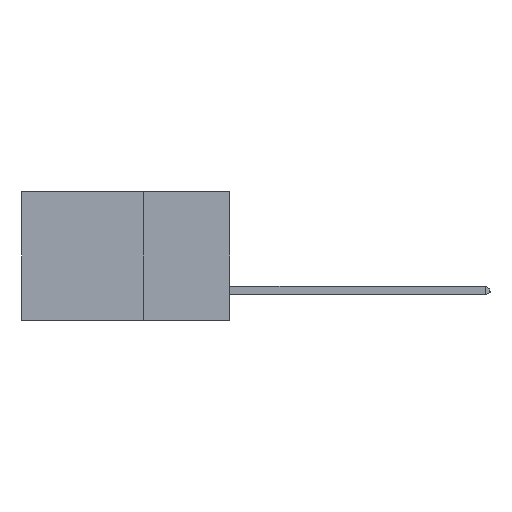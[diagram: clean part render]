
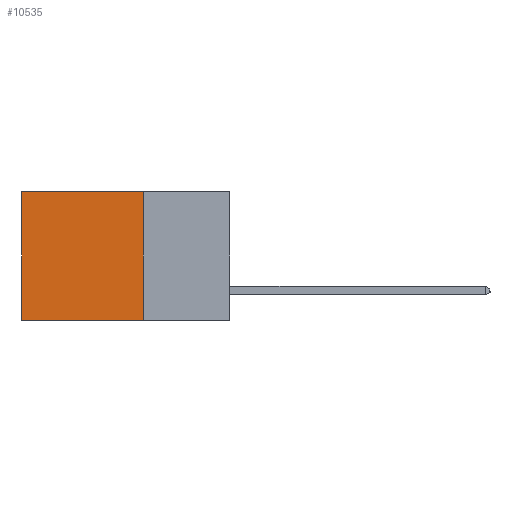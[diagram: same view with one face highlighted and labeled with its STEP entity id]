
A CAD part, left-side view. The second image highlights one B-rep face of the part: STEP entity #10535.
In plain terms, the highlighted planar face has unit normal (-1, 0, 0).
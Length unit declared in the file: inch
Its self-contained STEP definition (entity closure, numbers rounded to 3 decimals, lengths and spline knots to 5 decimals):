
#464 = EDGE_LOOP ( 'NONE', ( #13719, #4646, #3250, #9922 ) ) ;
#524 = FACE_OUTER_BOUND ( 'NONE', #464, .T. ) ;
#589 = VECTOR ( 'NONE', #6460, 39.37008 ) ;
#2047 = DIRECTION ( 'NONE',  ( 0., 0., -1. ) ) ;
#2952 = VECTOR ( 'NONE', #4228, 39.37008 ) ;
#3250 = ORIENTED_EDGE ( 'NONE', *, *, #14426, .F. ) ;
#4017 = CARTESIAN_POINT ( 'NONE',  ( 0.298, 0.6, 0. ) ) ;
#4228 = DIRECTION ( 'NONE',  ( 0., 0., -1. ) ) ;
#4241 = AXIS2_PLACEMENT_3D ( 'NONE', #12076, #4856, #4911 ) ;
#4599 = EDGE_CURVE ( 'NONE', #9386, #11939, #8337, .T. ) ;
#4646 = ORIENTED_EDGE ( 'NONE', *, *, #4599, .F. ) ;
#4856 = DIRECTION ( 'NONE',  ( 1., 0., 0. ) ) ;
#4911 = DIRECTION ( 'NONE',  ( 0., 0., -1. ) ) ;
#5129 = LINE ( 'NONE', #14431, #7232 ) ;
#5830 = DIRECTION ( 'NONE',  ( 0., 1., 0. ) ) ;
#6460 = DIRECTION ( 'NONE',  ( 0., 1., 0. ) ) ;
#7232 = VECTOR ( 'NONE', #5830, 39.37008 ) ;
#7370 = EDGE_CURVE ( 'NONE', #13046, #11939, #10689, .T. ) ;
#7529 = VERTEX_POINT ( 'NONE', #8713 ) ;
#8191 = CARTESIAN_POINT ( 'NONE',  ( 0.298, 0.25, -0.37 ) ) ;
#8337 = LINE ( 'NONE', #9948, #589 ) ;
#8713 = CARTESIAN_POINT ( 'NONE',  ( 0.298, 0.25, 0. ) ) ;
#9386 = VERTEX_POINT ( 'NONE', #8191 ) ;
#9922 = ORIENTED_EDGE ( 'NONE', *, *, #12759, .T. ) ;
#9948 = CARTESIAN_POINT ( 'NONE',  ( 0.298, 0.25, -0.37 ) ) ;
#10535 = ADVANCED_FACE ( 'NONE', ( #524 ), #10881, .F. ) ;
#10689 = LINE ( 'NONE', #12667, #2952 ) ;
#10881 = PLANE ( 'NONE',  #4241 ) ;
#11939 = VERTEX_POINT ( 'NONE', #14391 ) ;
#12076 = CARTESIAN_POINT ( 'NONE',  ( 0.298, 0.25, 0. ) ) ;
#12260 = VECTOR ( 'NONE', #2047, 39.37008 ) ;
#12667 = CARTESIAN_POINT ( 'NONE',  ( 0.298, 0.6, 0. ) ) ;
#12759 = EDGE_CURVE ( 'NONE', #7529, #13046, #5129, .T. ) ;
#13046 = VERTEX_POINT ( 'NONE', #4017 ) ;
#13212 = LINE ( 'NONE', #15161, #12260 ) ;
#13719 = ORIENTED_EDGE ( 'NONE', *, *, #7370, .T. ) ;
#14391 = CARTESIAN_POINT ( 'NONE',  ( 0.298, 0.6, -0.37 ) ) ;
#14426 = EDGE_CURVE ( 'NONE', #7529, #9386, #13212, .T. ) ;
#14431 = CARTESIAN_POINT ( 'NONE',  ( 0.298, 0.25, 0. ) ) ;
#15161 = CARTESIAN_POINT ( 'NONE',  ( 0.298, 0.25, 0. ) ) ;
